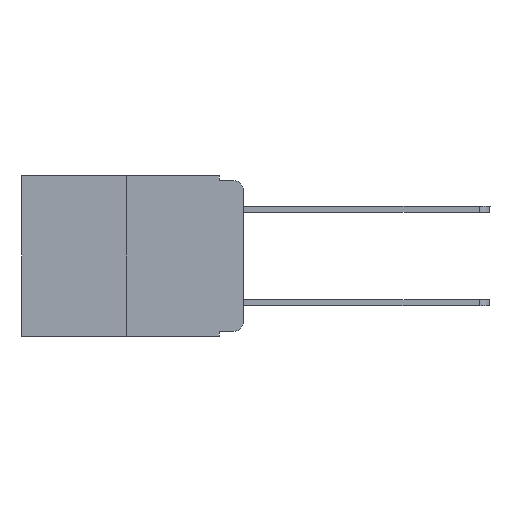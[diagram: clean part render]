
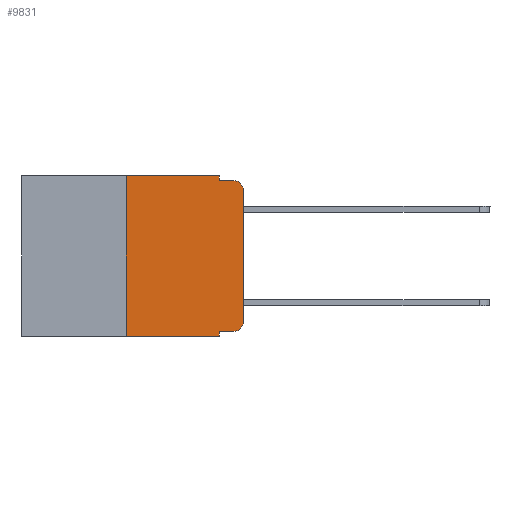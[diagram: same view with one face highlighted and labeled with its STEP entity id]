
A CAD part, left-side view. The second image highlights one B-rep face of the part: STEP entity #9831.
In plain terms, the highlighted planar face has unit normal (-1, 0, 0).
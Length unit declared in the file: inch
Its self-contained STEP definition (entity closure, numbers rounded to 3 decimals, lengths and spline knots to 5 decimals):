
#32 = AXIS2_PLACEMENT_3D ( 'NONE', #9378, #22058, #3333 ) ;
#466 = CARTESIAN_POINT ( 'NONE',  ( 0., 0.473, -0.343 ) ) ;
#679 = VECTOR ( 'NONE', #23664, 39.37008 ) ;
#885 = DIRECTION ( 'NONE',  ( 0., 0., -1. ) ) ;
#1389 = ORIENTED_EDGE ( 'NONE', *, *, #18425, .F. ) ;
#1505 = ORIENTED_EDGE ( 'NONE', *, *, #11709, .T. ) ;
#2029 = CARTESIAN_POINT ( 'NONE',  ( 0., 0., 0. ) ) ;
#2607 = CARTESIAN_POINT ( 'NONE',  ( 0., 0.051, -0.01 ) ) ;
#2852 = DIRECTION ( 'NONE',  ( 0., 0., -1. ) ) ;
#3234 = CARTESIAN_POINT ( 'NONE',  ( 0., 0.02, -0.03 ) ) ;
#3329 = EDGE_LOOP ( 'NONE', ( #17697, #4566, #25595, #19069, #24542, #9338, #14336, #1389, #1505, #11029 ) ) ;
#3333 = DIRECTION ( 'NONE',  ( 0., 0., -1. ) ) ;
#4334 = VECTOR ( 'NONE', #22797, 39.37008 ) ;
#4394 = CARTESIAN_POINT ( 'NONE',  ( 0., 0.02, -0.333 ) ) ;
#4498 = CARTESIAN_POINT ( 'NONE',  ( 0., 0.25, -0.343 ) ) ;
#4543 = VERTEX_POINT ( 'NONE', #16947 ) ;
#4566 = ORIENTED_EDGE ( 'NONE', *, *, #11691, .T. ) ;
#4954 = CARTESIAN_POINT ( 'NONE',  ( 0., 0.051, 0. ) ) ;
#5193 = DIRECTION ( 'NONE',  ( 1., 0., 0. ) ) ;
#5862 = CARTESIAN_POINT ( 'NONE',  ( 0., 0.25, 0. ) ) ;
#6117 = DIRECTION ( 'NONE',  ( 0., -1., 0. ) ) ;
#7046 = CARTESIAN_POINT ( 'NONE',  ( 0., 0.051, 0. ) ) ;
#7069 = DIRECTION ( 'NONE',  ( 0., -1., 0. ) ) ;
#7243 = PLANE ( 'NONE',  #10707 ) ;
#8021 = VERTEX_POINT ( 'NONE', #17216 ) ;
#8289 = VERTEX_POINT ( 'NONE', #25103 ) ;
#8778 = CIRCLE ( 'NONE', #32, 0.02 ) ;
#9087 = CIRCLE ( 'NONE', #22613, 0.02 ) ;
#9338 = ORIENTED_EDGE ( 'NONE', *, *, #15077, .F. ) ;
#9378 = CARTESIAN_POINT ( 'NONE',  ( 0., 0.02, -0.313 ) ) ;
#9617 = VERTEX_POINT ( 'NONE', #24604 ) ;
#9622 = VERTEX_POINT ( 'NONE', #4498 ) ;
#9638 = EDGE_CURVE ( 'NONE', #24639, #8289, #23216, .T. ) ;
#9831 = ADVANCED_FACE ( 'NONE', ( #13253 ), #7243, .F. ) ;
#10127 = VECTOR ( 'NONE', #12983, 39.37008 ) ;
#10707 = AXIS2_PLACEMENT_3D ( 'NONE', #21578, #5193, #2852 ) ;
#10988 = VECTOR ( 'NONE', #11902, 39.37008 ) ;
#11029 = ORIENTED_EDGE ( 'NONE', *, *, #26500, .T. ) ;
#11285 = CARTESIAN_POINT ( 'NONE',  ( 0., 0., -0.03 ) ) ;
#11374 = LINE ( 'NONE', #4954, #679 ) ;
#11494 = VECTOR ( 'NONE', #885, 39.37008 ) ;
#11596 = DIRECTION ( 'NONE',  ( -1., 0., 0. ) ) ;
#11691 = EDGE_CURVE ( 'NONE', #26474, #13141, #9087, .T. ) ;
#11709 = EDGE_CURVE ( 'NONE', #9617, #21391, #23745, .T. ) ;
#11902 = DIRECTION ( 'NONE',  ( 0., 0., 1. ) ) ;
#11905 = CARTESIAN_POINT ( 'NONE',  ( 0., 0.02, -0.01 ) ) ;
#12295 = LINE ( 'NONE', #13913, #24245 ) ;
#12983 = DIRECTION ( 'NONE',  ( 0., -1., 0. ) ) ;
#13141 = VERTEX_POINT ( 'NONE', #11905 ) ;
#13253 = FACE_OUTER_BOUND ( 'NONE', #3329, .T. ) ;
#13297 = EDGE_CURVE ( 'NONE', #8021, #26474, #20353, .T. ) ;
#13913 = CARTESIAN_POINT ( 'NONE',  ( 0., 0.051, -0.01 ) ) ;
#14070 = LINE ( 'NONE', #5862, #10988 ) ;
#14336 = ORIENTED_EDGE ( 'NONE', *, *, #17038, .T. ) ;
#14744 = VECTOR ( 'NONE', #7069, 39.37008 ) ;
#15077 = EDGE_CURVE ( 'NONE', #9622, #24639, #14070, .T. ) ;
#15092 = DIRECTION ( 'NONE',  ( 0., -1., 0. ) ) ;
#15665 = CARTESIAN_POINT ( 'NONE',  ( 0., 0.051, -0.333 ) ) ;
#16947 = CARTESIAN_POINT ( 'NONE',  ( 0., 0.051, -0.343 ) ) ;
#17038 = EDGE_CURVE ( 'NONE', #9622, #4543, #25346, .T. ) ;
#17216 = CARTESIAN_POINT ( 'NONE',  ( 0., 0., -0.313 ) ) ;
#17697 = ORIENTED_EDGE ( 'NONE', *, *, #13297, .T. ) ;
#17830 = CARTESIAN_POINT ( 'NONE',  ( 0., 0.25, 0. ) ) ;
#18425 = EDGE_CURVE ( 'NONE', #9617, #4543, #19452, .T. ) ;
#18970 = CARTESIAN_POINT ( 'NONE',  ( 0., 0.473, 0. ) ) ;
#19069 = ORIENTED_EDGE ( 'NONE', *, *, #21419, .F. ) ;
#19452 = LINE ( 'NONE', #7046, #11494 ) ;
#20353 = LINE ( 'NONE', #2029, #4334 ) ;
#21391 = VERTEX_POINT ( 'NONE', #4394 ) ;
#21419 = EDGE_CURVE ( 'NONE', #8289, #24970, #11374, .T. ) ;
#21552 = DIRECTION ( 'NONE',  ( 0., 0., -1. ) ) ;
#21578 = CARTESIAN_POINT ( 'NONE',  ( 0., 0.473, 0. ) ) ;
#22058 = DIRECTION ( 'NONE',  ( -1., 0., 0. ) ) ;
#22067 = EDGE_CURVE ( 'NONE', #24970, #13141, #12295, .T. ) ;
#22613 = AXIS2_PLACEMENT_3D ( 'NONE', #3234, #11596, #21552 ) ;
#22761 = VECTOR ( 'NONE', #15092, 39.37008 ) ;
#22797 = DIRECTION ( 'NONE',  ( 0., 0., 1. ) ) ;
#23216 = LINE ( 'NONE', #18970, #10127 ) ;
#23664 = DIRECTION ( 'NONE',  ( 0., 0., -1. ) ) ;
#23745 = LINE ( 'NONE', #15665, #14744 ) ;
#24245 = VECTOR ( 'NONE', #6117, 39.37008 ) ;
#24542 = ORIENTED_EDGE ( 'NONE', *, *, #9638, .F. ) ;
#24604 = CARTESIAN_POINT ( 'NONE',  ( 0., 0.051, -0.333 ) ) ;
#24639 = VERTEX_POINT ( 'NONE', #17830 ) ;
#24970 = VERTEX_POINT ( 'NONE', #2607 ) ;
#25103 = CARTESIAN_POINT ( 'NONE',  ( 0., 0.051, 0. ) ) ;
#25346 = LINE ( 'NONE', #466, #22761 ) ;
#25595 = ORIENTED_EDGE ( 'NONE', *, *, #22067, .F. ) ;
#26474 = VERTEX_POINT ( 'NONE', #11285 ) ;
#26500 = EDGE_CURVE ( 'NONE', #21391, #8021, #8778, .T. ) ;
